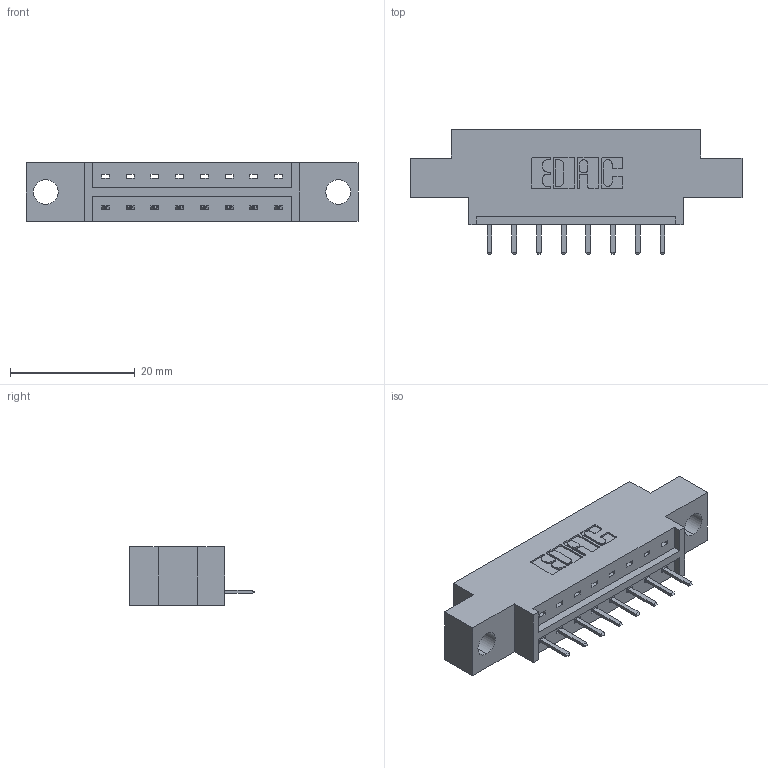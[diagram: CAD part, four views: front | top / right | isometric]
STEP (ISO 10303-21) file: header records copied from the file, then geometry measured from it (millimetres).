
FILE_DESCRIPTION (( 'STEP AP203' ), '1' );
FILE_NAME ('333-008-520-604.STEP', '2018-07-31T21:55:13', ( '' ), ( '' ), 'SwSTEP 2.0', 'SolidWorks 2016', '' );
FILE_SCHEMA (( 'CONFIG_CONTROL_DESIGN' ));
Length unit declared in the file: inch
Products named in the file (3): 345-292-001_345-293-120; 333-008-520-604; 333 Part_Offset - .156 Dia - TH
Assembly tree (9 placements, depth 2):
  333-008-520-604
    333 Part_Offset - .156 Dia - TH
    345-292-001_345-293-120  x8
Bounding box: 53.24 x 20.02 x 9.4 mm (x, y, z)
Volume: 4726.2 mm3; surface area: 4803.8 mm2
Topology: 9 solids, 9 shells, 614 faces, 1795 edges, 1174 vertices
Faces by surface type: plane 426, cylinder 188
Entity records: 9537 total; most frequent: CARTESIAN_POINT 1670, ORIENTED_EDGE 1602, DIRECTION 1465, EDGE_CURVE 801, LINE 669, VECTOR 669, VERTEX_POINT 530, AXIS2_PLACEMENT_3D 398
